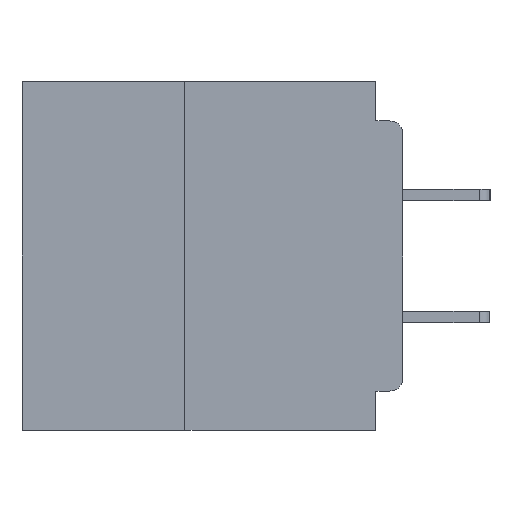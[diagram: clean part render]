
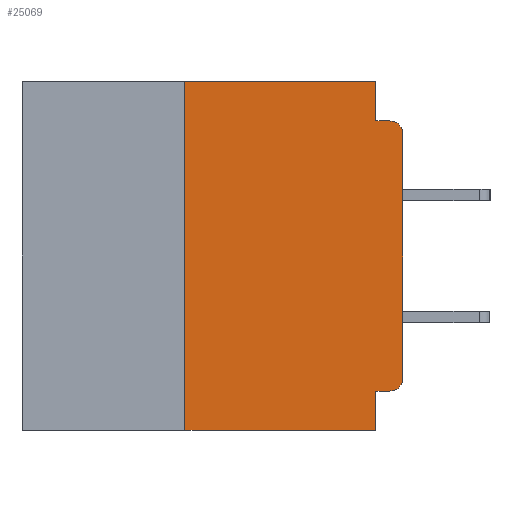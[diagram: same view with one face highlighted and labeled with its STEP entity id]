
A CAD part, left-side view. The second image highlights one B-rep face of the part: STEP entity #25069.
In plain terms, the highlighted planar face has unit normal (-1, 0, 0).
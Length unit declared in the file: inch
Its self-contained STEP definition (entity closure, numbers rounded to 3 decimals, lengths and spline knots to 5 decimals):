
#36 = LINE ( 'NONE', #47052, #19024 ) ;
#245 = VECTOR ( 'NONE', #14781, 39.37008 ) ;
#1852 = ORIENTED_EDGE ( 'NONE', *, *, #39731, .T. ) ;
#2268 = EDGE_CURVE ( 'NONE', #35484, #42537, #36, .T. ) ;
#2292 = VERTEX_POINT ( 'NONE', #10347 ) ;
#3640 = VERTEX_POINT ( 'NONE', #25301 ) ;
#4124 = DIRECTION ( 'NONE',  ( -1., 0., 0. ) ) ;
#5423 = AXIS2_PLACEMENT_3D ( 'NONE', #28297, #4124, #32290 ) ;
#5467 = VECTOR ( 'NONE', #40495, 39.37008 ) ;
#7415 = VERTEX_POINT ( 'NONE', #28160 ) ;
#9347 = EDGE_CURVE ( 'NONE', #13931, #35484, #47266, .T. ) ;
#9998 = EDGE_LOOP ( 'NONE', ( #44794, #1852, #27668, #20226, #18039, #28305, #39661, #12211, #11910, #21364 ) ) ;
#10347 = CARTESIAN_POINT ( 'NONE',  ( 0., 0.031, -0.355 ) ) ;
#10593 = CARTESIAN_POINT ( 'NONE',  ( 0., 0.25, 0. ) ) ;
#11910 = ORIENTED_EDGE ( 'NONE', *, *, #22508, .F. ) ;
#12211 = ORIENTED_EDGE ( 'NONE', *, *, #32802, .F. ) ;
#12296 = LINE ( 'NONE', #42701, #245 ) ;
#13057 = DIRECTION ( 'NONE',  ( 0., 0., 1. ) ) ;
#13791 = CARTESIAN_POINT ( 'NONE',  ( 0., 0.031, -0.045 ) ) ;
#13931 = VERTEX_POINT ( 'NONE', #36055 ) ;
#14126 = VERTEX_POINT ( 'NONE', #21424 ) ;
#14781 = DIRECTION ( 'NONE',  ( 0., -1., 0. ) ) ;
#15760 = EDGE_CURVE ( 'NONE', #35958, #22949, #42379, .T. ) ;
#16625 = CARTESIAN_POINT ( 'NONE',  ( 0., 0., -0.045 ) ) ;
#17441 = VECTOR ( 'NONE', #49852, 39.37008 ) ;
#17563 = LINE ( 'NONE', #16625, #5467 ) ;
#18039 = ORIENTED_EDGE ( 'NONE', *, *, #50162, .F. ) ;
#19012 = CARTESIAN_POINT ( 'NONE',  ( 0., 0.437, 0. ) ) ;
#19024 = VECTOR ( 'NONE', #13057, 39.37008 ) ;
#19652 = EDGE_CURVE ( 'NONE', #14126, #7415, #37373, .T. ) ;
#20226 = ORIENTED_EDGE ( 'NONE', *, *, #15760, .F. ) ;
#20230 = LINE ( 'NONE', #42962, #50739 ) ;
#21364 = ORIENTED_EDGE ( 'NONE', *, *, #9347, .T. ) ;
#21424 = CARTESIAN_POINT ( 'NONE',  ( 0., 0.25, -0.4 ) ) ;
#21997 = DIRECTION ( 'NONE',  ( 0., 0., -1. ) ) ;
#22012 = CARTESIAN_POINT ( 'NONE',  ( 0., 0.437, -0.4 ) ) ;
#22178 = CIRCLE ( 'NONE', #5423, 0.015 ) ;
#22444 = CARTESIAN_POINT ( 'NONE',  ( 0., 0.031, 0. ) ) ;
#22455 = VECTOR ( 'NONE', #21997, 39.37008 ) ;
#22508 = EDGE_CURVE ( 'NONE', #13931, #2292, #20230, .T. ) ;
#22869 = DIRECTION ( 'NONE',  ( -1., 0., 0. ) ) ;
#22949 = VERTEX_POINT ( 'NONE', #13791 ) ;
#23034 = PLANE ( 'NONE',  #46530 ) ;
#25069 = ADVANCED_FACE ( 'NONE', ( #34624 ), #23034, .F. ) ;
#25301 = CARTESIAN_POINT ( 'NONE',  ( 0., 0.015, -0.045 ) ) ;
#27051 = CARTESIAN_POINT ( 'NONE',  ( 0., 0.25, -0.4 ) ) ;
#27059 = DIRECTION ( 'NONE',  ( 0., 0., -1. ) ) ;
#27668 = ORIENTED_EDGE ( 'NONE', *, *, #28145, .F. ) ;
#28145 = EDGE_CURVE ( 'NONE', #22949, #3640, #17563, .T. ) ;
#28160 = CARTESIAN_POINT ( 'NONE',  ( 0., 0.031, -0.4 ) ) ;
#28297 = CARTESIAN_POINT ( 'NONE',  ( 0., 0.015, -0.06 ) ) ;
#28305 = ORIENTED_EDGE ( 'NONE', *, *, #50224, .F. ) ;
#28885 = DIRECTION ( 'NONE',  ( 0., 0., -1. ) ) ;
#31090 = VECTOR ( 'NONE', #28885, 39.37008 ) ;
#32290 = DIRECTION ( 'NONE',  ( 0., 0., -1. ) ) ;
#32802 = EDGE_CURVE ( 'NONE', #2292, #7415, #41686, .T. ) ;
#34624 = FACE_OUTER_BOUND ( 'NONE', #9998, .T. ) ;
#34686 = AXIS2_PLACEMENT_3D ( 'NONE', #46702, #22869, #50695 ) ;
#35484 = VERTEX_POINT ( 'NONE', #39526 ) ;
#35958 = VERTEX_POINT ( 'NONE', #22444 ) ;
#36055 = CARTESIAN_POINT ( 'NONE',  ( 0., 0.015, -0.355 ) ) ;
#37373 = LINE ( 'NONE', #22012, #17441 ) ;
#37921 = VECTOR ( 'NONE', #43031, 39.37008 ) ;
#38862 = DIRECTION ( 'NONE',  ( 1., 0., 0. ) ) ;
#39000 = VERTEX_POINT ( 'NONE', #10593 ) ;
#39171 = LINE ( 'NONE', #27051, #37921 ) ;
#39526 = CARTESIAN_POINT ( 'NONE',  ( 0., 0., -0.34 ) ) ;
#39661 = ORIENTED_EDGE ( 'NONE', *, *, #19652, .T. ) ;
#39731 = EDGE_CURVE ( 'NONE', #42537, #3640, #22178, .T. ) ;
#40495 = DIRECTION ( 'NONE',  ( 0., -1., 0. ) ) ;
#41686 = LINE ( 'NONE', #48864, #31090 ) ;
#42379 = LINE ( 'NONE', #45666, #22455 ) ;
#42537 = VERTEX_POINT ( 'NONE', #49404 ) ;
#42701 = CARTESIAN_POINT ( 'NONE',  ( 0., 0.437, 0. ) ) ;
#42962 = CARTESIAN_POINT ( 'NONE',  ( 0., 0., -0.355 ) ) ;
#43031 = DIRECTION ( 'NONE',  ( 0., 0., 1. ) ) ;
#44794 = ORIENTED_EDGE ( 'NONE', *, *, #2268, .T. ) ;
#45666 = CARTESIAN_POINT ( 'NONE',  ( 0., 0.031, 0. ) ) ;
#46530 = AXIS2_PLACEMENT_3D ( 'NONE', #19012, #38862, #27059 ) ;
#46702 = CARTESIAN_POINT ( 'NONE',  ( 0., 0.015, -0.34 ) ) ;
#46975 = DIRECTION ( 'NONE',  ( 0., 1., 0. ) ) ;
#47052 = CARTESIAN_POINT ( 'NONE',  ( 0., 0., 0. ) ) ;
#47266 = CIRCLE ( 'NONE', #34686, 0.015 ) ;
#48864 = CARTESIAN_POINT ( 'NONE',  ( 0., 0.031, -0.4 ) ) ;
#49404 = CARTESIAN_POINT ( 'NONE',  ( 0., 0., -0.06 ) ) ;
#49852 = DIRECTION ( 'NONE',  ( 0., -1., 0. ) ) ;
#50162 = EDGE_CURVE ( 'NONE', #39000, #35958, #12296, .T. ) ;
#50224 = EDGE_CURVE ( 'NONE', #14126, #39000, #39171, .T. ) ;
#50695 = DIRECTION ( 'NONE',  ( 0., 0., -1. ) ) ;
#50739 = VECTOR ( 'NONE', #46975, 39.37008 ) ;
